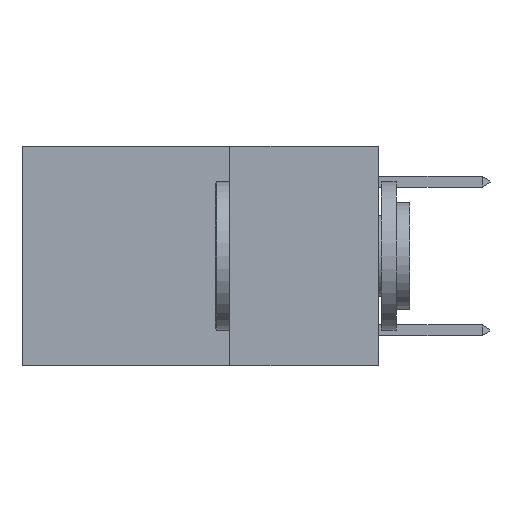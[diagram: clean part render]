
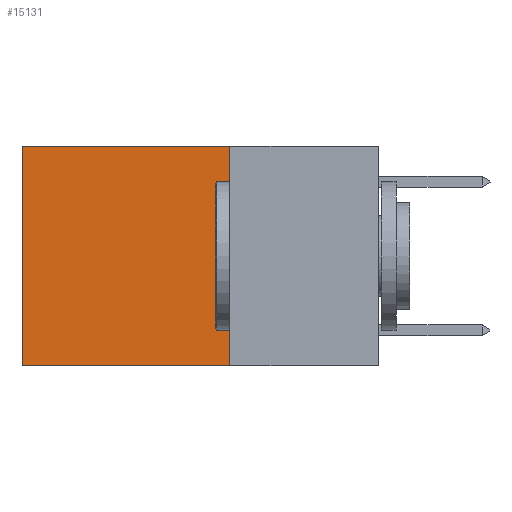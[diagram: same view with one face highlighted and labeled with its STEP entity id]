
A CAD part, left-side view. The second image highlights one B-rep face of the part: STEP entity #15131.
In plain terms, the highlighted planar face has unit normal (-1, 0, 0).
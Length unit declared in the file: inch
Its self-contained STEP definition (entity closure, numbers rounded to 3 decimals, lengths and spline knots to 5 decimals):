
#102 = CARTESIAN_POINT ( 'NONE',  ( 0.2625, 0.25, 0. ) ) ;
#200 = LINE ( 'NONE', #102, #17339 ) ;
#1163 = VERTEX_POINT ( 'NONE', #15353 ) ;
#2196 = PLANE ( 'NONE',  #7507 ) ;
#2282 = LINE ( 'NONE', #7761, #2471 ) ;
#2471 = VECTOR ( 'NONE', #11720, 39.37008 ) ;
#3185 = EDGE_CURVE ( 'NONE', #11048, #12705, #16572, .T. ) ;
#3608 = CARTESIAN_POINT ( 'NONE',  ( 0.2625, 0.25, 0. ) ) ;
#5798 = CARTESIAN_POINT ( 'NONE',  ( 0.2625, 0.25, 0. ) ) ;
#5846 = LINE ( 'NONE', #14001, #9725 ) ;
#6020 = DIRECTION ( 'NONE',  ( 0., 1., 0. ) ) ;
#6555 = ORIENTED_EDGE ( 'NONE', *, *, #9556, .F. ) ;
#7443 = VECTOR ( 'NONE', #9844, 39.37008 ) ;
#7507 = AXIS2_PLACEMENT_3D ( 'NONE', #11563, #14253, #7591 ) ;
#7591 = DIRECTION ( 'NONE',  ( 0., 0., -1. ) ) ;
#7761 = CARTESIAN_POINT ( 'NONE',  ( 0.2625, 0.6, 0. ) ) ;
#8408 = EDGE_LOOP ( 'NONE', ( #14562, #6555, #15025, #16155 ) ) ;
#9556 = EDGE_CURVE ( 'NONE', #13834, #1163, #5846, .T. ) ;
#9725 = VECTOR ( 'NONE', #6020, 39.37008 ) ;
#9745 = DIRECTION ( 'NONE',  ( 0., 0., -1. ) ) ;
#9844 = DIRECTION ( 'NONE',  ( 0., 1., 0. ) ) ;
#10736 = CARTESIAN_POINT ( 'NONE',  ( 0.2625, 0.25, -0.37 ) ) ;
#11048 = VERTEX_POINT ( 'NONE', #3608 ) ;
#11563 = CARTESIAN_POINT ( 'NONE',  ( 0.2625, 0.25, 0. ) ) ;
#11625 = EDGE_CURVE ( 'NONE', #12705, #1163, #2282, .T. ) ;
#11720 = DIRECTION ( 'NONE',  ( 0., 0., -1. ) ) ;
#12705 = VERTEX_POINT ( 'NONE', #16367 ) ;
#13834 = VERTEX_POINT ( 'NONE', #10736 ) ;
#14001 = CARTESIAN_POINT ( 'NONE',  ( 0.2625, 0.25, -0.37 ) ) ;
#14253 = DIRECTION ( 'NONE',  ( 1., 0., 0. ) ) ;
#14562 = ORIENTED_EDGE ( 'NONE', *, *, #11625, .T. ) ;
#15025 = ORIENTED_EDGE ( 'NONE', *, *, #17228, .F. ) ;
#15131 = ADVANCED_FACE ( 'NONE', ( #15701 ), #2196, .F. ) ;
#15353 = CARTESIAN_POINT ( 'NONE',  ( 0.2625, 0.6, -0.37 ) ) ;
#15701 = FACE_OUTER_BOUND ( 'NONE', #8408, .T. ) ;
#16155 = ORIENTED_EDGE ( 'NONE', *, *, #3185, .T. ) ;
#16367 = CARTESIAN_POINT ( 'NONE',  ( 0.2625, 0.6, 0. ) ) ;
#16572 = LINE ( 'NONE', #5798, #7443 ) ;
#17228 = EDGE_CURVE ( 'NONE', #11048, #13834, #200, .T. ) ;
#17339 = VECTOR ( 'NONE', #9745, 39.37008 ) ;
